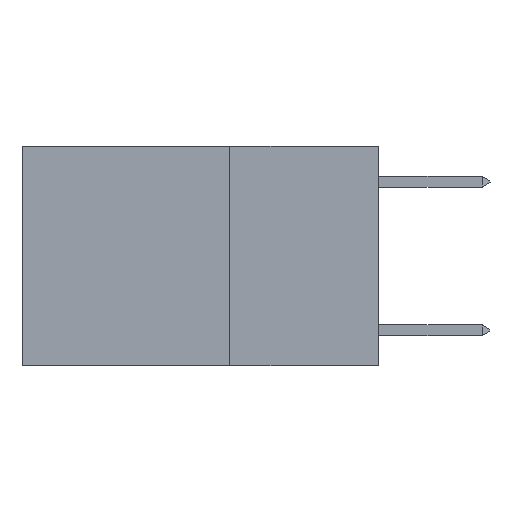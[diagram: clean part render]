
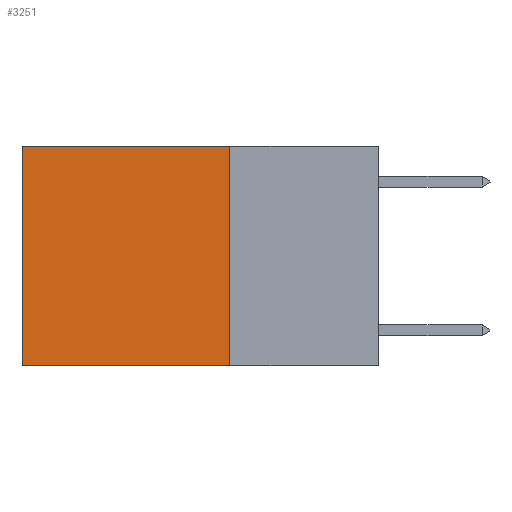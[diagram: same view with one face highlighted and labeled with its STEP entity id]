
A CAD part, left-side view. The second image highlights one B-rep face of the part: STEP entity #3251.
In plain terms, the highlighted planar face has unit normal (-1, 0, 0).
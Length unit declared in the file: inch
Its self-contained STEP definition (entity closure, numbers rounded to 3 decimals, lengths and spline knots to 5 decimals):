
#314 = CARTESIAN_POINT ( 'NONE',  ( 0.2625, 0.25, 0. ) ) ;
#2057 = DIRECTION ( 'NONE',  ( 0., 0., -1. ) ) ;
#2571 = VERTEX_POINT ( 'NONE', #14781 ) ;
#3251 = ADVANCED_FACE ( 'NONE', ( #16889 ), #5947, .F. ) ;
#3253 = LINE ( 'NONE', #4341, #4083 ) ;
#4083 = VECTOR ( 'NONE', #11099, 39.37008 ) ;
#4178 = CARTESIAN_POINT ( 'NONE',  ( 0.2625, 0.25, 0. ) ) ;
#4334 = LINE ( 'NONE', #9814, #8226 ) ;
#4341 = CARTESIAN_POINT ( 'NONE',  ( 0.2625, 0.25, 0. ) ) ;
#4713 = AXIS2_PLACEMENT_3D ( 'NONE', #4178, #9665, #15283 ) ;
#5284 = ORIENTED_EDGE ( 'NONE', *, *, #10110, .F. ) ;
#5664 = VECTOR ( 'NONE', #2057, 39.37008 ) ;
#5667 = VECTOR ( 'NONE', #15489, 39.37008 ) ;
#5702 = CARTESIAN_POINT ( 'NONE',  ( 0.2625, 0.25, -0.37 ) ) ;
#5772 = VERTEX_POINT ( 'NONE', #16582 ) ;
#5947 = PLANE ( 'NONE',  #4713 ) ;
#6040 = EDGE_CURVE ( 'NONE', #2571, #5772, #14290, .T. ) ;
#7334 = CARTESIAN_POINT ( 'NONE',  ( 0.2625, 0.6, 0. ) ) ;
#8207 = EDGE_LOOP ( 'NONE', ( #10147, #16496, #5284, #15354 ) ) ;
#8226 = VECTOR ( 'NONE', #16852, 39.37008 ) ;
#8410 = LINE ( 'NONE', #5702, #5667 ) ;
#8509 = VERTEX_POINT ( 'NONE', #9042 ) ;
#9042 = CARTESIAN_POINT ( 'NONE',  ( 0.2625, 0.25, -0.37 ) ) ;
#9665 = DIRECTION ( 'NONE',  ( 1., 0., 0. ) ) ;
#9814 = CARTESIAN_POINT ( 'NONE',  ( 0.2625, 0.25, 0. ) ) ;
#10110 = EDGE_CURVE ( 'NONE', #15695, #8509, #3253, .T. ) ;
#10147 = ORIENTED_EDGE ( 'NONE', *, *, #6040, .T. ) ;
#10438 = EDGE_CURVE ( 'NONE', #8509, #5772, #8410, .T. ) ;
#11099 = DIRECTION ( 'NONE',  ( 0., 0., -1. ) ) ;
#14290 = LINE ( 'NONE', #7334, #5664 ) ;
#14781 = CARTESIAN_POINT ( 'NONE',  ( 0.2625, 0.6, 0. ) ) ;
#15283 = DIRECTION ( 'NONE',  ( 0., 0., -1. ) ) ;
#15354 = ORIENTED_EDGE ( 'NONE', *, *, #16209, .T. ) ;
#15489 = DIRECTION ( 'NONE',  ( 0., 1., 0. ) ) ;
#15695 = VERTEX_POINT ( 'NONE', #314 ) ;
#16209 = EDGE_CURVE ( 'NONE', #15695, #2571, #4334, .T. ) ;
#16496 = ORIENTED_EDGE ( 'NONE', *, *, #10438, .F. ) ;
#16582 = CARTESIAN_POINT ( 'NONE',  ( 0.2625, 0.6, -0.37 ) ) ;
#16852 = DIRECTION ( 'NONE',  ( 0., 1., 0. ) ) ;
#16889 = FACE_OUTER_BOUND ( 'NONE', #8207, .T. ) ;
